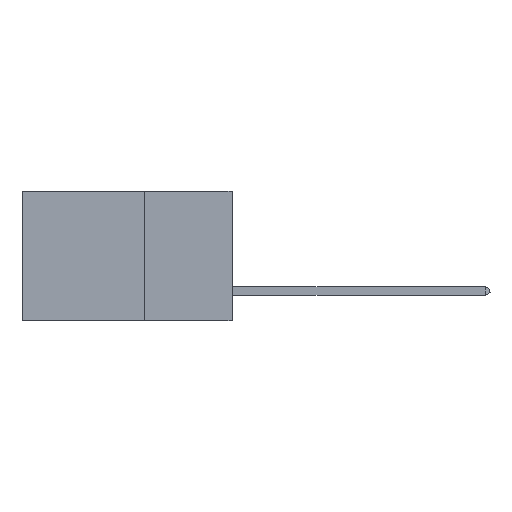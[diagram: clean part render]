
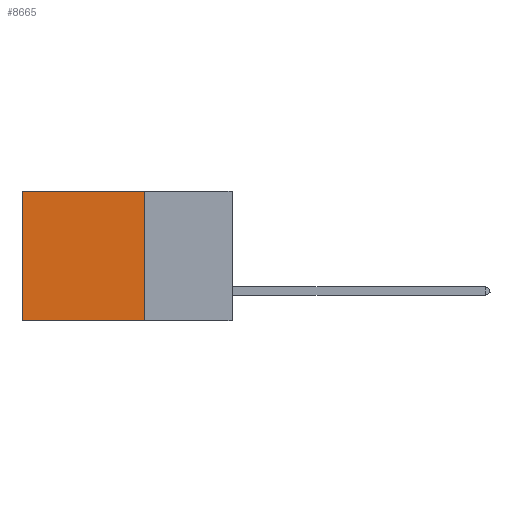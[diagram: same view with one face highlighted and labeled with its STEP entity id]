
A CAD part, left-side view. The second image highlights one B-rep face of the part: STEP entity #8665.
In plain terms, the highlighted planar face has unit normal (-1, 0, 0).
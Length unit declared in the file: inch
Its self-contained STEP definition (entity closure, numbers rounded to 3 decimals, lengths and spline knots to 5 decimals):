
#1241 = EDGE_CURVE ( 'NONE', #18769, #32886, #30407, .T. ) ;
#1379 = LINE ( 'NONE', #23944, #30333 ) ;
#1727 = DIRECTION ( 'NONE',  ( 0., 0., -1. ) ) ;
#1872 = CARTESIAN_POINT ( 'NONE',  ( 0.2875, 0.25, -0.37 ) ) ;
#2019 = ORIENTED_EDGE ( 'NONE', *, *, #9261, .F. ) ;
#2187 = CARTESIAN_POINT ( 'NONE',  ( 0.2875, 0.25, -0.37 ) ) ;
#2616 = LINE ( 'NONE', #1872, #20637 ) ;
#4639 = ORIENTED_EDGE ( 'NONE', *, *, #7076, .F. ) ;
#5066 = DIRECTION ( 'NONE',  ( 0., 0., -1. ) ) ;
#6716 = EDGE_CURVE ( 'NONE', #32886, #28002, #11455, .T. ) ;
#7076 = EDGE_CURVE ( 'NONE', #18769, #20469, #1379, .T. ) ;
#8054 = ORIENTED_EDGE ( 'NONE', *, *, #1241, .T. ) ;
#8665 = ADVANCED_FACE ( 'NONE', ( #13460 ), #28250, .F. ) ;
#8969 = CARTESIAN_POINT ( 'NONE',  ( 0.2875, 0.6, 0. ) ) ;
#9261 = EDGE_CURVE ( 'NONE', #20469, #28002, #2616, .T. ) ;
#11455 = LINE ( 'NONE', #24638, #12748 ) ;
#12748 = VECTOR ( 'NONE', #27200, 39.37008 ) ;
#13178 = ORIENTED_EDGE ( 'NONE', *, *, #6716, .T. ) ;
#13460 = FACE_OUTER_BOUND ( 'NONE', #23904, .T. ) ;
#14929 = VECTOR ( 'NONE', #24279, 39.37008 ) ;
#18769 = VERTEX_POINT ( 'NONE', #32806 ) ;
#20254 = CARTESIAN_POINT ( 'NONE',  ( 0.2875, 0.25, 0. ) ) ;
#20469 = VERTEX_POINT ( 'NONE', #2187 ) ;
#20637 = VECTOR ( 'NONE', #23132, 39.37008 ) ;
#22564 = CARTESIAN_POINT ( 'NONE',  ( 0.2875, 0.6, -0.37 ) ) ;
#23132 = DIRECTION ( 'NONE',  ( 0., 1., 0. ) ) ;
#23822 = AXIS2_PLACEMENT_3D ( 'NONE', #20254, #27762, #1727 ) ;
#23904 = EDGE_LOOP ( 'NONE', ( #13178, #2019, #4639, #8054 ) ) ;
#23944 = CARTESIAN_POINT ( 'NONE',  ( 0.2875, 0.25, 0. ) ) ;
#24279 = DIRECTION ( 'NONE',  ( 0., 1., 0. ) ) ;
#24638 = CARTESIAN_POINT ( 'NONE',  ( 0.2875, 0.6, 0. ) ) ;
#27200 = DIRECTION ( 'NONE',  ( 0., 0., -1. ) ) ;
#27762 = DIRECTION ( 'NONE',  ( 1., 0., 0. ) ) ;
#28002 = VERTEX_POINT ( 'NONE', #22564 ) ;
#28250 = PLANE ( 'NONE',  #23822 ) ;
#29400 = CARTESIAN_POINT ( 'NONE',  ( 0.2875, 0.25, 0. ) ) ;
#30333 = VECTOR ( 'NONE', #5066, 39.37008 ) ;
#30407 = LINE ( 'NONE', #29400, #14929 ) ;
#32806 = CARTESIAN_POINT ( 'NONE',  ( 0.2875, 0.25, 0. ) ) ;
#32886 = VERTEX_POINT ( 'NONE', #8969 ) ;
